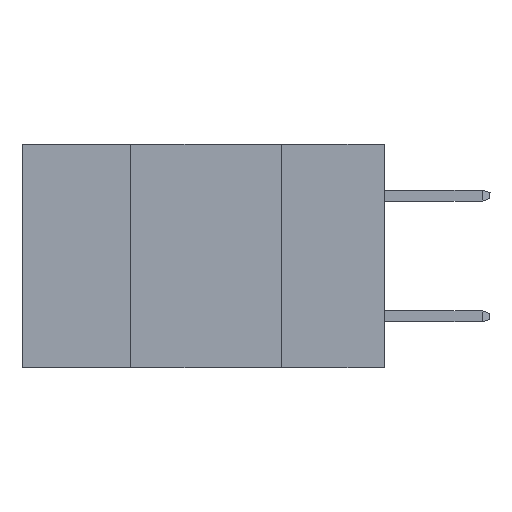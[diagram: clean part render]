
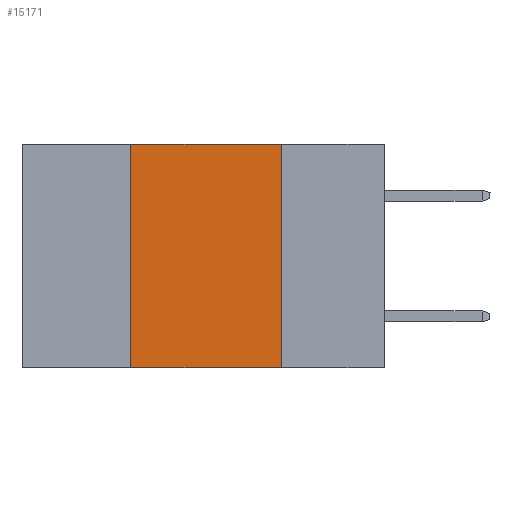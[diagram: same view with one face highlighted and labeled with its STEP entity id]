
A CAD part, left-side view. The second image highlights one B-rep face of the part: STEP entity #15171.
In plain terms, the highlighted planar face has unit normal (-1, 0, 0).
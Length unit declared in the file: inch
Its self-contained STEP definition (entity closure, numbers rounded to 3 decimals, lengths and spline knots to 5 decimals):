
#1054 = PLANE ( 'NONE',  #14160 ) ;
#1847 = CARTESIAN_POINT ( 'NONE',  ( 0., 0.42, -0.37 ) ) ;
#2837 = ORIENTED_EDGE ( 'NONE', *, *, #7746, .T. ) ;
#3835 = VECTOR ( 'NONE', #26544, 39.37008 ) ;
#4243 = LINE ( 'NONE', #4317, #12099 ) ;
#4317 = CARTESIAN_POINT ( 'NONE',  ( 0., 0.17, 0. ) ) ;
#4422 = CARTESIAN_POINT ( 'NONE',  ( 0., 0.6, -0.37 ) ) ;
#4616 = VERTEX_POINT ( 'NONE', #1847 ) ;
#6158 = EDGE_CURVE ( 'NONE', #4616, #33725, #24546, .T. ) ;
#7020 = DIRECTION ( 'NONE',  ( 0., 0., -1. ) ) ;
#7693 = VERTEX_POINT ( 'NONE', #9551 ) ;
#7746 = EDGE_CURVE ( 'NONE', #4616, #7693, #10206, .T. ) ;
#9551 = CARTESIAN_POINT ( 'NONE',  ( 0., 0.17, -0.37 ) ) ;
#9705 = EDGE_CURVE ( 'NONE', #26490, #7693, #4243, .T. ) ;
#10206 = LINE ( 'NONE', #4422, #23177 ) ;
#10560 = CARTESIAN_POINT ( 'NONE',  ( 0., 0.17, 0. ) ) ;
#11100 = ORIENTED_EDGE ( 'NONE', *, *, #6158, .F. ) ;
#11778 = CARTESIAN_POINT ( 'NONE',  ( 0., 0.6, 0. ) ) ;
#12099 = VECTOR ( 'NONE', #7020, 39.37008 ) ;
#14160 = AXIS2_PLACEMENT_3D ( 'NONE', #11778, #29921, #14389 ) ;
#14389 = DIRECTION ( 'NONE',  ( 0., 0., -1. ) ) ;
#15171 = ADVANCED_FACE ( 'NONE', ( #26063 ), #1054, .F. ) ;
#16115 = ORIENTED_EDGE ( 'NONE', *, *, #16410, .F. ) ;
#16410 = EDGE_CURVE ( 'NONE', #33725, #26490, #24711, .T. ) ;
#17648 = VECTOR ( 'NONE', #26731, 39.37008 ) ;
#19709 = ORIENTED_EDGE ( 'NONE', *, *, #9705, .F. ) ;
#22679 = DIRECTION ( 'NONE',  ( 0., -1., 0. ) ) ;
#23177 = VECTOR ( 'NONE', #22679, 39.37008 ) ;
#23924 = CARTESIAN_POINT ( 'NONE',  ( 0., 0.6, 0. ) ) ;
#24546 = LINE ( 'NONE', #26801, #17648 ) ;
#24711 = LINE ( 'NONE', #23924, #3835 ) ;
#26063 = FACE_OUTER_BOUND ( 'NONE', #27774, .T. ) ;
#26490 = VERTEX_POINT ( 'NONE', #10560 ) ;
#26544 = DIRECTION ( 'NONE',  ( 0., -1., 0. ) ) ;
#26731 = DIRECTION ( 'NONE',  ( 0., 0., 1. ) ) ;
#26801 = CARTESIAN_POINT ( 'NONE',  ( 0., 0.42, 0. ) ) ;
#27774 = EDGE_LOOP ( 'NONE', ( #19709, #16115, #11100, #2837 ) ) ;
#29921 = DIRECTION ( 'NONE',  ( 1., 0., 0. ) ) ;
#32684 = CARTESIAN_POINT ( 'NONE',  ( 0., 0.42, 0. ) ) ;
#33725 = VERTEX_POINT ( 'NONE', #32684 ) ;
